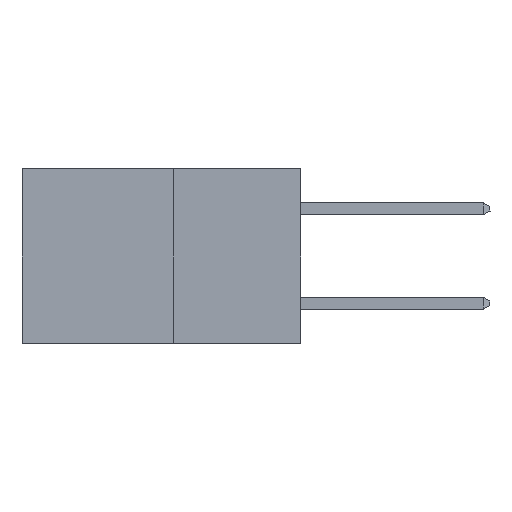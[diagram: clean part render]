
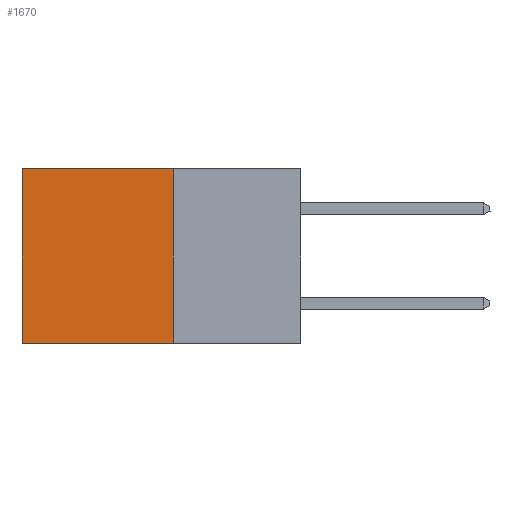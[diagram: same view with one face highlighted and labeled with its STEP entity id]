
A CAD part, left-side view. The second image highlights one B-rep face of the part: STEP entity #1670.
In plain terms, the highlighted planar face has unit normal (-1, 0, 0).
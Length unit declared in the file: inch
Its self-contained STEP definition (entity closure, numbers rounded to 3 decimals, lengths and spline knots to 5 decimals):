
#319 = VECTOR ( 'NONE', #18683, 39.37008 ) ;
#1043 = LINE ( 'NONE', #9758, #319 ) ;
#1670 = ADVANCED_FACE ( 'NONE', ( #1770 ), #21310, .F. ) ;
#1770 = FACE_OUTER_BOUND ( 'NONE', #9062, .T. ) ;
#2120 = CARTESIAN_POINT ( 'NONE',  ( 0.277, 0.27, -0.37 ) ) ;
#2541 = CARTESIAN_POINT ( 'NONE',  ( 0.277, 0.59, -0.37 ) ) ;
#2814 = ORIENTED_EDGE ( 'NONE', *, *, #24622, .T. ) ;
#3799 = ORIENTED_EDGE ( 'NONE', *, *, #10255, .T. ) ;
#4253 = DIRECTION ( 'NONE',  ( 0., 1., 0. ) ) ;
#4578 = VERTEX_POINT ( 'NONE', #15695 ) ;
#4736 = VECTOR ( 'NONE', #4253, 39.37008 ) ;
#5532 = CARTESIAN_POINT ( 'NONE',  ( 0.277, 0.27, -0.37 ) ) ;
#7437 = VERTEX_POINT ( 'NONE', #2541 ) ;
#8390 = CARTESIAN_POINT ( 'NONE',  ( 0.277, 0.59, -0.37 ) ) ;
#9062 = EDGE_LOOP ( 'NONE', ( #2814, #18079, #16458, #3799 ) ) ;
#9758 = CARTESIAN_POINT ( 'NONE',  ( 0.277, 0.27, -0.37 ) ) ;
#10200 = VERTEX_POINT ( 'NONE', #15374 ) ;
#10255 = EDGE_CURVE ( 'NONE', #26992, #4578, #16779, .T. ) ;
#10931 = DIRECTION ( 'NONE',  ( 0., 0., -1. ) ) ;
#11802 = AXIS2_PLACEMENT_3D ( 'NONE', #2120, #19832, #10931 ) ;
#11877 = VECTOR ( 'NONE', #27862, 39.37008 ) ;
#12583 = LINE ( 'NONE', #5532, #11877 ) ;
#15374 = CARTESIAN_POINT ( 'NONE',  ( 0.277, 0.27, -0.37 ) ) ;
#15695 = CARTESIAN_POINT ( 'NONE',  ( 0.277, 0.59, 0. ) ) ;
#16264 = EDGE_CURVE ( 'NONE', #10200, #7437, #12583, .T. ) ;
#16458 = ORIENTED_EDGE ( 'NONE', *, *, #17624, .F. ) ;
#16779 = LINE ( 'NONE', #17708, #4736 ) ;
#17574 = CARTESIAN_POINT ( 'NONE',  ( 0.277, 0.27, 0. ) ) ;
#17624 = EDGE_CURVE ( 'NONE', #26992, #10200, #1043, .T. ) ;
#17708 = CARTESIAN_POINT ( 'NONE',  ( 0.277, 0.27, 0. ) ) ;
#18079 = ORIENTED_EDGE ( 'NONE', *, *, #16264, .F. ) ;
#18683 = DIRECTION ( 'NONE',  ( 0., 0., -1. ) ) ;
#19832 = DIRECTION ( 'NONE',  ( 1., 0., 0. ) ) ;
#21310 = PLANE ( 'NONE',  #11802 ) ;
#21846 = DIRECTION ( 'NONE',  ( 0., 0., -1. ) ) ;
#23801 = VECTOR ( 'NONE', #21846, 39.37008 ) ;
#24622 = EDGE_CURVE ( 'NONE', #4578, #7437, #28925, .T. ) ;
#26992 = VERTEX_POINT ( 'NONE', #17574 ) ;
#27862 = DIRECTION ( 'NONE',  ( 0., 1., 0. ) ) ;
#28925 = LINE ( 'NONE', #8390, #23801 ) ;
